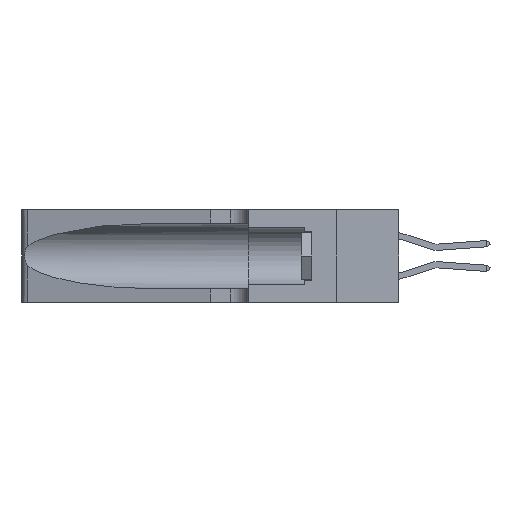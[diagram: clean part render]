
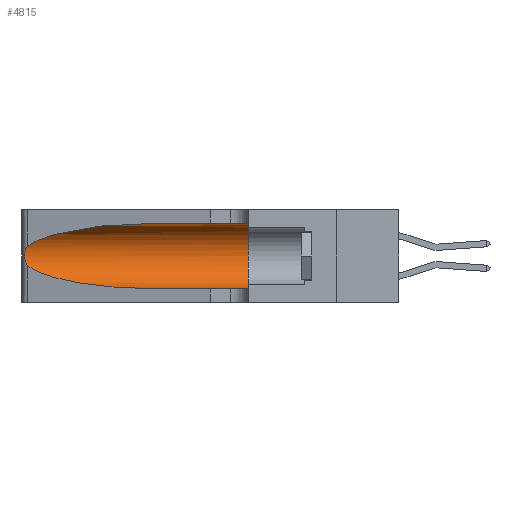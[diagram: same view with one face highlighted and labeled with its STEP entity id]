
A CAD part, left-side view. The second image highlights one B-rep face of the part: STEP entity #4815.
In plain terms, the highlighted cylindrical face has radius 3.308 mm (diameter 6.617 mm), a partial arc.
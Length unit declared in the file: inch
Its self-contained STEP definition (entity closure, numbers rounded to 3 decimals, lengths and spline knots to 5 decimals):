
#540 = CARTESIAN_POINT ( 'NONE',  ( 0.2373, 1.15595, 0.08982 ) ) ;
#576 = DIRECTION ( 'NONE',  ( 0., -1., 0. ) ) ;
#611 = CARTESIAN_POINT ( 'NONE',  ( 0.1305, 0.35, 0.05475 ) ) ;
#1997 = ORIENTED_EDGE ( 'NONE', *, *, #24537, .T. ) ;
#2220 = CARTESIAN_POINT ( 'NONE',  ( 0.25555, 1.22993, 0.14849 ) ) ;
#2450 = LINE ( 'NONE', #25354, #9518 ) ;
#2825 = CARTESIAN_POINT ( 'NONE',  ( 0.25487, 1.22718, 0.14631 ) ) ;
#2995 = CYLINDRICAL_SURFACE ( 'NONE', #14640, 0.13025 ) ;
#3287 =( BOUNDED_CURVE ( )  B_SPLINE_CURVE ( 3, ( #2825, #540, #5310, #22084 ),
 .UNSPECIFIED., .F., .F. ) 
 B_SPLINE_CURVE_WITH_KNOTS ( ( 4, 4 ),
 ( 3.44316, 4.71239 ),
 .UNSPECIFIED. ) 
 CURVE ( )  GEOMETRIC_REPRESENTATION_ITEM ( )  RATIONAL_B_SPLINE_CURVE ( ( 1., 0.87, 0.87, 1. ) ) 
 REPRESENTATION_ITEM ( '' )  );
#4311 = ORIENTED_EDGE ( 'NONE', *, *, #14448, .F. ) ;
#4509 = CARTESIAN_POINT ( 'NONE',  ( 0.25487, 1.22718, 0.22369 ) ) ;
#4815 = ADVANCED_FACE ( 'NONE', ( #22087 ), #2995, .F. ) ;
#4824 = CARTESIAN_POINT ( 'NONE',  ( 0.25487, 1.22718, 0.14631 ) ) ;
#5270 = VERTEX_POINT ( 'NONE', #15529 ) ;
#5310 = CARTESIAN_POINT ( 'NONE',  ( 0.18966, 0.96281, 0.05475 ) ) ;
#5517 = EDGE_CURVE ( 'NONE', #5270, #25902, #16058, .T. ) ;
#5530 = EDGE_CURVE ( 'NONE', #13370, #22768, #27649, .T. ) ;
#5626 = EDGE_LOOP ( 'NONE', ( #1997, #11741, #19669, #29219, #14183, #4311 ) ) ;
#6050 = LINE ( 'NONE', #12449, #29737 ) ;
#6905 = CARTESIAN_POINT ( 'NONE',  ( 0.25787, 1.23484, 0.2124 ) ) ;
#9306 = CARTESIAN_POINT ( 'NONE',  ( 0.26018, 1.23835, 0.19895 ) ) ;
#9325 = CARTESIAN_POINT ( 'NONE',  ( 0.2373, 1.15595, 0.28018 ) ) ;
#9518 = VECTOR ( 'NONE', #11086, 39.37008 ) ;
#10304 = CARTESIAN_POINT ( 'NONE',  ( 0.1305, 0.72297, 0.31525 ) ) ;
#11086 = DIRECTION ( 'NONE',  ( 0., -1., 0. ) ) ;
#11566 = EDGE_CURVE ( 'NONE', #12798, #25902, #2450, .T. ) ;
#11601 = CARTESIAN_POINT ( 'NONE',  ( 0.25555, 1.22994, 0.2215 ) ) ;
#11703 = CARTESIAN_POINT ( 'NONE',  ( 0.26075, 1.23896, 0.178 ) ) ;
#11741 = ORIENTED_EDGE ( 'NONE', *, *, #5530, .T. ) ;
#12449 = CARTESIAN_POINT ( 'NONE',  ( 0.1305, 1.61858, 0.31525 ) ) ;
#12798 = VERTEX_POINT ( 'NONE', #21187 ) ;
#13370 = VERTEX_POINT ( 'NONE', #18523 ) ;
#14050 = CARTESIAN_POINT ( 'NONE',  ( 0.1305, 0.35, 0.185 ) ) ;
#14147 = CARTESIAN_POINT ( 'NONE',  ( 0.25856, 1.23593, 0.16098 ) ) ;
#14183 = ORIENTED_EDGE ( 'NONE', *, *, #5517, .F. ) ;
#14418 =( BOUNDED_CURVE ( )  B_SPLINE_CURVE ( 3, ( #21205, #21307, #9325, #25958 ),
 .UNSPECIFIED., .F., .F. ) 
 B_SPLINE_CURVE_WITH_KNOTS ( ( 4, 4 ),
 ( 1.5708, 2.84003 ),
 .UNSPECIFIED. ) 
 CURVE ( )  GEOMETRIC_REPRESENTATION_ITEM ( )  RATIONAL_B_SPLINE_CURVE ( ( 1., 0.87, 0.87, 1. ) ) 
 REPRESENTATION_ITEM ( '' )  );
#14448 = EDGE_CURVE ( 'NONE', #25263, #5270, #6050, .T. ) ;
#14640 = AXIS2_PLACEMENT_3D ( 'NONE', #21014, #16193, #18596 ) ;
#15529 = CARTESIAN_POINT ( 'NONE',  ( 0.1305, 0.35, 0.31525 ) ) ;
#16058 = CIRCLE ( 'NONE', #24610, 0.13025 ) ;
#16193 = DIRECTION ( 'NONE',  ( 0., -1., 0. ) ) ;
#16457 = DIRECTION ( 'NONE',  ( 0., 0., 1. ) ) ;
#16574 = CARTESIAN_POINT ( 'NONE',  ( 0.25639, 1.23186, 0.15144 ) ) ;
#18523 = CARTESIAN_POINT ( 'NONE',  ( 0.25487, 1.22718, 0.22369 ) ) ;
#18596 = DIRECTION ( 'NONE',  ( 0., 0., -1. ) ) ;
#18969 = CARTESIAN_POINT ( 'NONE',  ( 0.25487, 1.22718, 0.14631 ) ) ;
#19669 = ORIENTED_EDGE ( 'NONE', *, *, #29828, .T. ) ;
#21014 = CARTESIAN_POINT ( 'NONE',  ( 0.1305, 1.61858, 0.185 ) ) ;
#21187 = CARTESIAN_POINT ( 'NONE',  ( 0.1305, 0.72297, 0.05475 ) ) ;
#21205 = CARTESIAN_POINT ( 'NONE',  ( 0.1305, 0.72297, 0.31525 ) ) ;
#21307 = CARTESIAN_POINT ( 'NONE',  ( 0.18966, 0.96281, 0.31525 ) ) ;
#22084 = CARTESIAN_POINT ( 'NONE',  ( 0.1305, 0.72297, 0.05475 ) ) ;
#22087 = FACE_OUTER_BOUND ( 'NONE', #5626, .T. ) ;
#22768 = VERTEX_POINT ( 'NONE', #4824 ) ;
#23650 = CARTESIAN_POINT ( 'NONE',  ( 0.25854, 1.2359, 0.20912 ) ) ;
#24537 = EDGE_CURVE ( 'NONE', #25263, #13370, #14418, .T. ) ;
#24610 = AXIS2_PLACEMENT_3D ( 'NONE', #14050, #30499, #16457 ) ;
#25263 = VERTEX_POINT ( 'NONE', #10304 ) ;
#25354 = CARTESIAN_POINT ( 'NONE',  ( 0.1305, 1.61858, 0.05475 ) ) ;
#25844 = CARTESIAN_POINT ( 'NONE',  ( 0.25639, 1.23184, 0.21858 ) ) ;
#25902 = VERTEX_POINT ( 'NONE', #611 ) ;
#25938 = CARTESIAN_POINT ( 'NONE',  ( 0.26075, 1.23896, 0.19203 ) ) ;
#25958 = CARTESIAN_POINT ( 'NONE',  ( 0.25487, 1.22718, 0.22369 ) ) ;
#27649 = B_SPLINE_CURVE_WITH_KNOTS ( 'NONE', 3,
 ( #4509, #11601, #25844, #6905, #23650, #9306, #25938, #11703, #28278, #14147, #30600, #16574, #2220, #18969 ),
 .UNSPECIFIED., .F., .F.,
 ( 4, 2, 2, 2, 2, 2, 4 ),
 ( 0., 0.00027, 0.00053, 0.00107, 0.0016, 0.00187, 0.00214 ),
 .UNSPECIFIED. ) ;
#28278 = CARTESIAN_POINT ( 'NONE',  ( 0.26017, 1.23833, 0.17102 ) ) ;
#29219 = ORIENTED_EDGE ( 'NONE', *, *, #11566, .T. ) ;
#29737 = VECTOR ( 'NONE', #576, 39.37008 ) ;
#29828 = EDGE_CURVE ( 'NONE', #22768, #12798, #3287, .T. ) ;
#30499 = DIRECTION ( 'NONE',  ( 0., 1., 0. ) ) ;
#30600 = CARTESIAN_POINT ( 'NONE',  ( 0.25789, 1.23486, 0.15765 ) ) ;
